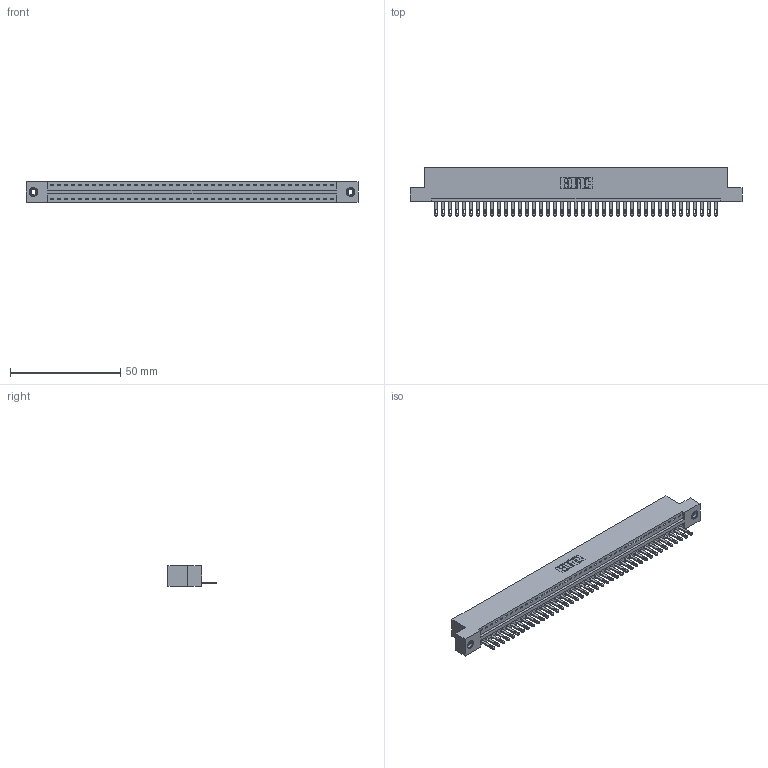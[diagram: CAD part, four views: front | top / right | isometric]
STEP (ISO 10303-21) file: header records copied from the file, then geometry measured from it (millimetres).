
FILE_DESCRIPTION (( 'STEP AP203' ), '1' );
FILE_NAME ('346-041-500-108.STEP', '2018-08-24T10:58:34', ( '' ), ( '' ), 'SwSTEP 2.0', 'SolidWorks 2016', '' );
FILE_SCHEMA (( 'CONFIG_CONTROL_DESIGN' ));
Length unit declared in the file: inch
Products named in the file (4): 346 Part_Flush Mounting Lugs - 0.156 Dia-TI; 345-292-001_345-293-100; 345-250-001_345-250-003-102; 346-041-500-108
Assembly tree (44 placements, depth 2):
  346-041-500-108
    346 Part_Flush Mounting Lugs - 0.156 Dia-TI
    345-292-001_345-293-100  x41
    345-250-001_345-250-003-102  x2
Bounding box: 150.75 x 21.84 x 9.4 mm (x, y, z)
Volume: 14442 mm3; surface area: 18157.2 mm2
Topology: 44 solids, 44 shells, 2396 faces, 7353 edges, 4894 vertices
Faces by surface type: plane 1502, cylinder 878, cone 12, torus 4
Entity records: 26696 total; most frequent: CARTESIAN_POINT 4558, ORIENTED_EDGE 4526, DIRECTION 4051, EDGE_CURVE 2263, LINE 1943, VECTOR 1943, VERTEX_POINT 1504, AXIS2_PLACEMENT_3D 1054
